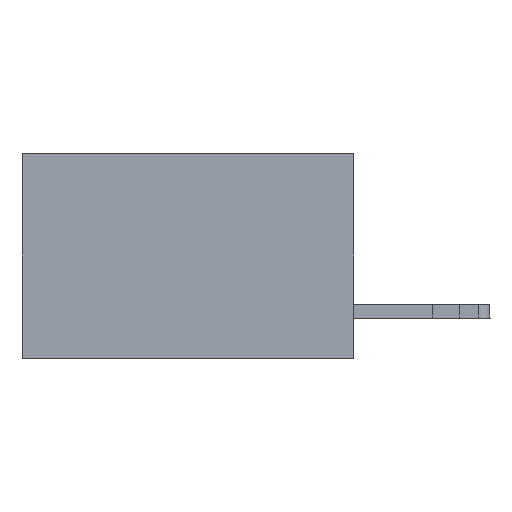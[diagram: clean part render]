
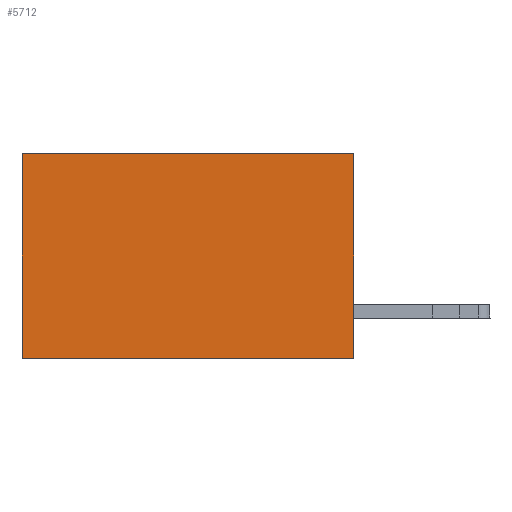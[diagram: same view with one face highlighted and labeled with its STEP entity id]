
A CAD part, left-side view. The second image highlights one B-rep face of the part: STEP entity #5712.
In plain terms, the highlighted planar face has unit normal (-1, 0, 0).
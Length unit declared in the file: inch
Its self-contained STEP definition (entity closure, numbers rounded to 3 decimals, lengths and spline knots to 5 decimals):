
#410 = ORIENTED_EDGE ( 'NONE', *, *, #2499, .F. ) ;
#2499 = EDGE_CURVE ( 'NONE', #21494, #22663, #6620, .T. ) ;
#4294 = DIRECTION ( 'NONE',  ( 0., 0., -1. ) ) ;
#4883 = CARTESIAN_POINT ( 'NONE',  ( 0.2875, 0.6, -0.37 ) ) ;
#5546 = ORIENTED_EDGE ( 'NONE', *, *, #29055, .T. ) ;
#5712 = ADVANCED_FACE ( 'NONE', ( #34566 ), #20376, .F. ) ;
#6180 = DIRECTION ( 'NONE',  ( 0., 0., -1. ) ) ;
#6290 = LINE ( 'NONE', #18239, #14857 ) ;
#6620 = LINE ( 'NONE', #16250, #13201 ) ;
#6622 = AXIS2_PLACEMENT_3D ( 'NONE', #13950, #23576, #4294 ) ;
#9283 = CARTESIAN_POINT ( 'NONE',  ( 0.2875, 0., 0. ) ) ;
#11160 = VECTOR ( 'NONE', #6180, 39.37008 ) ;
#12720 = ORIENTED_EDGE ( 'NONE', *, *, #16187, .T. ) ;
#13201 = VECTOR ( 'NONE', #28647, 39.37008 ) ;
#13950 = CARTESIAN_POINT ( 'NONE',  ( 0.2875, 0., 0. ) ) ;
#14182 = VERTEX_POINT ( 'NONE', #22073 ) ;
#14857 = VECTOR ( 'NONE', #39999, 39.37008 ) ;
#15343 = VERTEX_POINT ( 'NONE', #20408 ) ;
#16187 = EDGE_CURVE ( 'NONE', #14182, #15343, #6290, .T. ) ;
#16250 = CARTESIAN_POINT ( 'NONE',  ( 0.2875, 0., -0.37 ) ) ;
#18239 = CARTESIAN_POINT ( 'NONE',  ( 0.2875, 0., 0. ) ) ;
#19558 = EDGE_LOOP ( 'NONE', ( #5546, #410, #28524, #12720 ) ) ;
#20376 = PLANE ( 'NONE',  #6622 ) ;
#20408 = CARTESIAN_POINT ( 'NONE',  ( 0.2875, 0.6, 0. ) ) ;
#21494 = VERTEX_POINT ( 'NONE', #39991 ) ;
#22073 = CARTESIAN_POINT ( 'NONE',  ( 0.2875, 0., 0. ) ) ;
#22663 = VERTEX_POINT ( 'NONE', #4883 ) ;
#23576 = DIRECTION ( 'NONE',  ( 1., 0., 0. ) ) ;
#28403 = LINE ( 'NONE', #9283, #35638 ) ;
#28524 = ORIENTED_EDGE ( 'NONE', *, *, #29655, .F. ) ;
#28647 = DIRECTION ( 'NONE',  ( 0., 1., 0. ) ) ;
#29055 = EDGE_CURVE ( 'NONE', #15343, #22663, #36171, .T. ) ;
#29655 = EDGE_CURVE ( 'NONE', #14182, #21494, #28403, .T. ) ;
#31555 = CARTESIAN_POINT ( 'NONE',  ( 0.2875, 0.6, 0. ) ) ;
#34566 = FACE_OUTER_BOUND ( 'NONE', #19558, .T. ) ;
#35638 = VECTOR ( 'NONE', #37549, 39.37008 ) ;
#36171 = LINE ( 'NONE', #31555, #11160 ) ;
#37549 = DIRECTION ( 'NONE',  ( 0., 0., -1. ) ) ;
#39991 = CARTESIAN_POINT ( 'NONE',  ( 0.2875, 0., -0.37 ) ) ;
#39999 = DIRECTION ( 'NONE',  ( 0., 1., 0. ) ) ;
